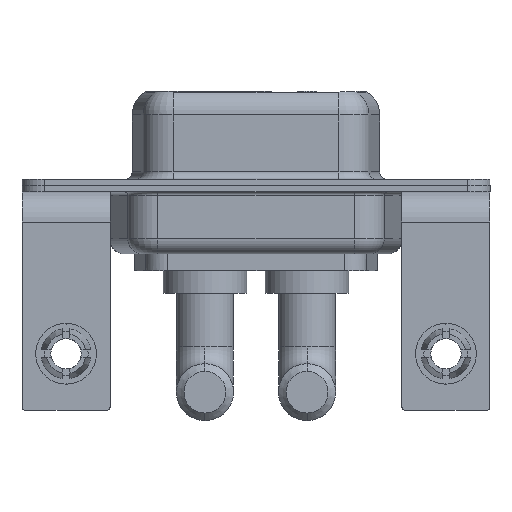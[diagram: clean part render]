
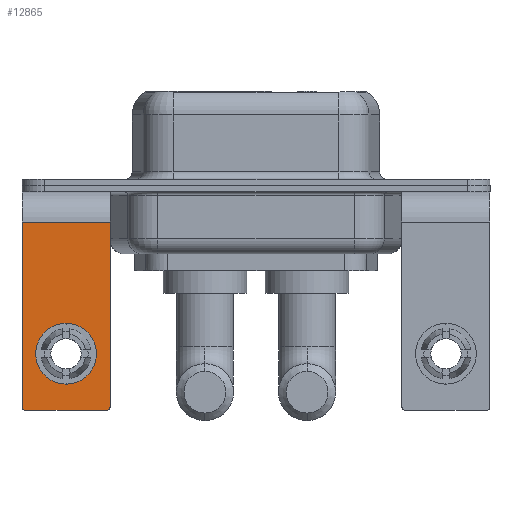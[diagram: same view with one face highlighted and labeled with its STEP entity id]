
A CAD part, front view. The second image highlights one B-rep face of the part: STEP entity #12865.
In plain terms, the highlighted planar face has unit normal (0, -1, 0).
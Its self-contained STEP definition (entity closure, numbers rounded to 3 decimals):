
#468 = CARTESIAN_POINT ( 'NONE',  ( -2.9, -6.25, -2.4 ) ) ;
#940 = ORIENTED_EDGE ( 'NONE', *, *, #9250, .F. ) ;
#1854 = FACE_OUTER_BOUND ( 'NONE', #3713, .T. ) ;
#1897 = ORIENTED_EDGE ( 'NONE', *, *, #9086, .T. ) ;
#1911 = EDGE_CURVE ( 'NONE', #5339, #12443, #13799, .T. ) ;
#1940 = DIRECTION ( 'NONE',  ( 0., 0., -1. ) ) ;
#2595 = VERTEX_POINT ( 'NONE', #468 ) ;
#2767 = CIRCLE ( 'NONE', #5292, 0.25 ) ;
#3001 = DIRECTION ( 'NONE',  ( 0., -1., 0. ) ) ;
#3013 = CARTESIAN_POINT ( 'NONE',  ( -2.9, -6.25, -2.4 ) ) ;
#3713 = EDGE_LOOP ( 'NONE', ( #4191, #1897, #9066, #11623, #940, #12482 ) ) ;
#3756 = CARTESIAN_POINT ( 'NONE',  ( 2.9, -6.25, -2.4 ) ) ;
#3996 = DIRECTION ( 'NONE',  ( 0., 0., 1. ) ) ;
#4020 = DIRECTION ( 'NONE',  ( 0., 0., 1. ) ) ;
#4109 = VERTEX_POINT ( 'NONE', #15315 ) ;
#4160 = AXIS2_PLACEMENT_3D ( 'NONE', #11465, #5418, #4229 ) ;
#4191 = ORIENTED_EDGE ( 'NONE', *, *, #8152, .T. ) ;
#4229 = DIRECTION ( 'NONE',  ( 0., 0., 1. ) ) ;
#4315 = DIRECTION ( 'NONE',  ( 0., 0., 1. ) ) ;
#4596 = AXIS2_PLACEMENT_3D ( 'NONE', #10199, #13676, #4315 ) ;
#4936 = EDGE_CURVE ( 'NONE', #7866, #10407, #2767, .T. ) ;
#5276 = CARTESIAN_POINT ( 'NONE',  ( 0., -6.25, -13.07 ) ) ;
#5292 = AXIS2_PLACEMENT_3D ( 'NONE', #15154, #3001, #4020 ) ;
#5339 = VERTEX_POINT ( 'NONE', #6459 ) ;
#5383 = ORIENTED_EDGE ( 'NONE', *, *, #1911, .T. ) ;
#5418 = DIRECTION ( 'NONE',  ( 0., 1., 0. ) ) ;
#5467 = LINE ( 'NONE', #3013, #9136 ) ;
#5834 = AXIS2_PLACEMENT_3D ( 'NONE', #13717, #12612, #11591 ) ;
#5849 = VECTOR ( 'NONE', #14091, 1000. ) ;
#6125 = LINE ( 'NONE', #9947, #13254 ) ;
#6369 = DIRECTION ( 'NONE',  ( 0., 1., 0. ) ) ;
#6450 = CARTESIAN_POINT ( 'NONE',  ( 0., -6.25, -11.07 ) ) ;
#6459 = CARTESIAN_POINT ( 'NONE',  ( 0., -6.25, -9.07 ) ) ;
#6597 = FACE_BOUND ( 'NONE', #12956, .T. ) ;
#6670 = PLANE ( 'NONE',  #4160 ) ;
#7129 = VECTOR ( 'NONE', #1940, 1000. ) ;
#7384 = CIRCLE ( 'NONE', #4596, 0.25 ) ;
#7866 = VERTEX_POINT ( 'NONE', #9309 ) ;
#8152 = EDGE_CURVE ( 'NONE', #2595, #13736, #5467, .T. ) ;
#8176 = EDGE_CURVE ( 'NONE', #12443, #5339, #15478, .T. ) ;
#8788 = EDGE_CURVE ( 'NONE', #7866, #4109, #13060, .T. ) ;
#8834 = CARTESIAN_POINT ( 'NONE',  ( 2.9, -6.25, -14.55 ) ) ;
#9066 = ORIENTED_EDGE ( 'NONE', *, *, #8788, .F. ) ;
#9086 = EDGE_CURVE ( 'NONE', #13736, #4109, #7384, .T. ) ;
#9136 = VECTOR ( 'NONE', #10466, 1000. ) ;
#9250 = EDGE_CURVE ( 'NONE', #14158, #10407, #11779, .T. ) ;
#9309 = CARTESIAN_POINT ( 'NONE',  ( 2.65, -6.25, -14.8 ) ) ;
#9947 = CARTESIAN_POINT ( 'NONE',  ( 2.9, -6.25, -2.4 ) ) ;
#10199 = CARTESIAN_POINT ( 'NONE',  ( -2.65, -6.25, -14.55 ) ) ;
#10261 = AXIS2_PLACEMENT_3D ( 'NONE', #6450, #6369, #3996 ) ;
#10407 = VERTEX_POINT ( 'NONE', #8834 ) ;
#10450 = CARTESIAN_POINT ( 'NONE',  ( 2.9, -6.25, -14.8 ) ) ;
#10466 = DIRECTION ( 'NONE',  ( 0., 0., -1. ) ) ;
#10764 = EDGE_CURVE ( 'NONE', #14158, #2595, #6125, .T. ) ;
#11465 = CARTESIAN_POINT ( 'NONE',  ( 2.9, -6.25, -2.4 ) ) ;
#11569 = CARTESIAN_POINT ( 'NONE',  ( -2.9, -6.25, -14.55 ) ) ;
#11591 = DIRECTION ( 'NONE',  ( 0., 0., 1. ) ) ;
#11623 = ORIENTED_EDGE ( 'NONE', *, *, #4936, .T. ) ;
#11779 = LINE ( 'NONE', #12819, #7129 ) ;
#12253 = DIRECTION ( 'NONE',  ( -1., 0., 0. ) ) ;
#12443 = VERTEX_POINT ( 'NONE', #5276 ) ;
#12482 = ORIENTED_EDGE ( 'NONE', *, *, #10764, .T. ) ;
#12612 = DIRECTION ( 'NONE',  ( 0., 1., 0. ) ) ;
#12785 = ORIENTED_EDGE ( 'NONE', *, *, #8176, .T. ) ;
#12819 = CARTESIAN_POINT ( 'NONE',  ( 2.9, -6.25, -2.4 ) ) ;
#12865 = ADVANCED_FACE ( 'NONE', ( #6597, #1854 ), #6670, .F. ) ;
#12956 = EDGE_LOOP ( 'NONE', ( #12785, #5383 ) ) ;
#13060 = LINE ( 'NONE', #10450, #5849 ) ;
#13254 = VECTOR ( 'NONE', #12253, 1000. ) ;
#13676 = DIRECTION ( 'NONE',  ( 0., -1., 0. ) ) ;
#13717 = CARTESIAN_POINT ( 'NONE',  ( 0., -6.25, -11.07 ) ) ;
#13736 = VERTEX_POINT ( 'NONE', #11569 ) ;
#13799 = CIRCLE ( 'NONE', #10261, 2. ) ;
#14091 = DIRECTION ( 'NONE',  ( -1., 0., 0. ) ) ;
#14158 = VERTEX_POINT ( 'NONE', #3756 ) ;
#15154 = CARTESIAN_POINT ( 'NONE',  ( 2.65, -6.25, -14.55 ) ) ;
#15315 = CARTESIAN_POINT ( 'NONE',  ( -2.65, -6.25, -14.8 ) ) ;
#15478 = CIRCLE ( 'NONE', #5834, 2. ) ;
